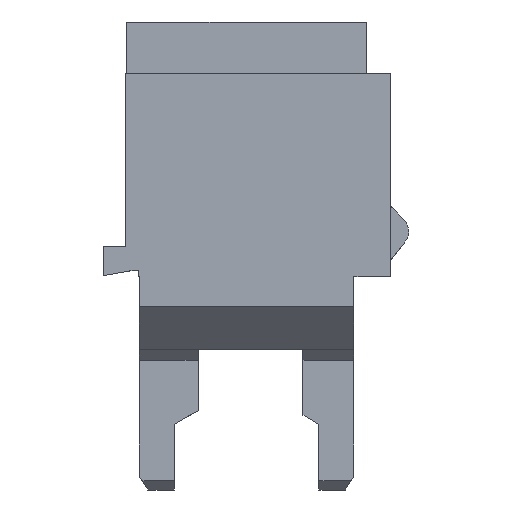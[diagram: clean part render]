
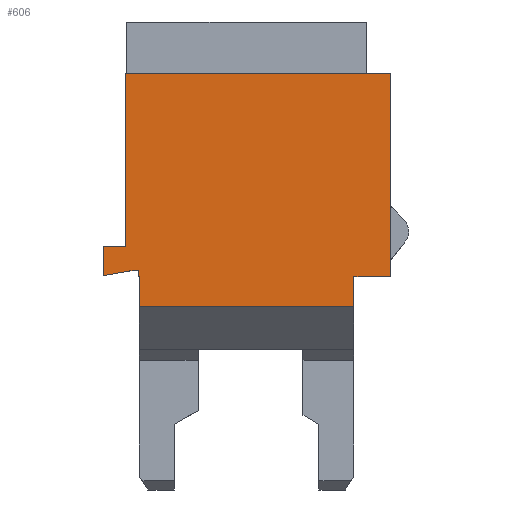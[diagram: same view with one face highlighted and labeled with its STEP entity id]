
A CAD part, left-side view. The second image highlights one B-rep face of the part: STEP entity #606.
In plain terms, the highlighted planar face has unit normal (-1, 0, 0).
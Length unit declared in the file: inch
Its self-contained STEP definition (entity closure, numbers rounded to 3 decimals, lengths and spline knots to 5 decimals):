
#606=ADVANCED_FACE('',(#1566),#1567,.T.);
#782=EDGE_CURVE('',#1823,#1816,#1826,.T.);
#816=EDGE_CURVE('',#1836,#1872,#1875,.T.);
#822=EDGE_CURVE('',#1880,#1872,#1883,.T.);
#858=EDGE_CURVE('',#1880,#1932,#1935,.T.);
#1100=EDGE_CURVE('',#2256,#2253,#2257,.T.);
#1106=EDGE_CURVE('',#2256,#2261,#2264,.T.);
#1136=EDGE_CURVE('',#2301,#1816,#2302,.T.);
#1138=EDGE_CURVE('',#2261,#1823,#2304,.T.);
#1140=EDGE_CURVE('',#2253,#2306,#2307,.T.);
#1142=EDGE_CURVE('',#2306,#2309,#2310,.T.);
#1144=EDGE_CURVE('',#2312,#2309,#2313,.T.);
#1146=EDGE_CURVE('',#1836,#2312,#2315,.T.);
#1148=EDGE_CURVE('',#2301,#1932,#2317,.T.);
#1566=FACE_OUTER_BOUND('',#2773,.T.);
#1567=PLANE('',#2774);
#1816=VERTEX_POINT('',#3138);
#1823=VERTEX_POINT('',#3149);
#1826=LINE('',#3154,#3155);
#1836=VERTEX_POINT('',#3169);
#1872=VERTEX_POINT('',#3227);
#1875=LINE('',#3232,#3233);
#1880=VERTEX_POINT('',#3241);
#1883=LINE('',#3246,#3247);
#1932=VERTEX_POINT('',#3327);
#1935=LINE('',#3332,#3333);
#2253=VERTEX_POINT('',#3877);
#2256=VERTEX_POINT('',#3882);
#2257=LINE('',#3883,#3884);
#2261=VERTEX_POINT('',#3891);
#2264=LINE('',#3896,#3897);
#2301=VERTEX_POINT('',#3962);
#2302=LINE('',#3963,#3964);
#2304=LINE('',#3967,#3968);
#2306=VERTEX_POINT('',#3971);
#2307=LINE('',#3972,#3973);
#2309=VERTEX_POINT('',#3976);
#2310=LINE('',#3977,#3978);
#2312=VERTEX_POINT('',#3981);
#2313=LINE('',#3982,#3983);
#2315=LINE('',#3986,#3987);
#2317=LINE('',#3990,#3991);
#2773=EDGE_LOOP('',(#5173,#5174,#5175,#5176,#5177,#5178,#5179,#5180,#5181,#5182,#5183,#5184,#5185));
#2774=AXIS2_PLACEMENT_3D('',#5186,#5187,#5188);
#3138=CARTESIAN_POINT('',(0.0,-0.0705,2.075));
#3149=CARTESIAN_POINT('',(0.0,1.4745,2.075));
#3154=CARTESIAN_POINT('',(0.0,-0.0555,2.075));
#3155=VECTOR('',#5633,0.03937);
#3169=CARTESIAN_POINT('',(0.0,1.395,0.89));
#3227=CARTESIAN_POINT('',(0.0,1.395,0.715));
#3232=CARTESIAN_POINT('',(0.0,1.395,0.71016));
#3233=VECTOR('',#5660,0.03937);
#3241=CARTESIAN_POINT('',(0.0,0.145,0.715));
#3246=CARTESIAN_POINT('',(0.0,1.614,0.715));
#3247=VECTOR('',#5663,0.03937);
#3327=CARTESIAN_POINT('',(0.0,0.145,0.89));
#3332=CARTESIAN_POINT('',(0.0,0.145,0.71016));
#3333=VECTOR('',#5685,0.03937);
#3877=CARTESIAN_POINT('',(0.0,1.6045,0.89553));
#3882=CARTESIAN_POINT('',(0.0,1.6045,1.068));
#3883=CARTESIAN_POINT('',(0.0,1.6045,1.44156));
#3884=VECTOR('',#5832,0.03937);
#3891=CARTESIAN_POINT('',(0.0,1.4745,1.068));
#3896=CARTESIAN_POINT('',(0.0,-0.00806,1.068));
#3897=VECTOR('',#5835,0.03937);
#3962=CARTESIAN_POINT('',(0.0,-0.0705,0.89));
#3963=CARTESIAN_POINT('',(0.0,-0.0705,1.45141));
#3964=VECTOR('',#5852,0.03937);
#3967=CARTESIAN_POINT('',(0.0,1.4745,1.19609));
#3968=VECTOR('',#5853,0.03937);
#3971=CARTESIAN_POINT('',(0.,1.44366,0.92389));
#3972=CARTESIAN_POINT('',(0.,0.72763,1.05014));
#3973=VECTOR('',#5854,0.03937);
#3976=CARTESIAN_POINT('',(0.,1.398,0.92389));
#3977=CARTESIAN_POINT('',(0.,1.44366,0.92389));
#3978=VECTOR('',#5855,0.03937);
#3981=CARTESIAN_POINT('',(0.0,1.398,0.89));
#3982=CARTESIAN_POINT('',(0.0,1.398,1.46125));
#3983=VECTOR('',#5856,0.03937);
#3986=CARTESIAN_POINT('',(0.0,1.6075,0.89));
#3987=VECTOR('',#5857,0.03937);
#3990=CARTESIAN_POINT('',(0.0,1.6075,0.89));
#3991=VECTOR('',#5858,0.03937);
#5173=ORIENTED_EDGE('',*,*,#1136,.T.);
#5174=ORIENTED_EDGE('',*,*,#782,.F.);
#5175=ORIENTED_EDGE('',*,*,#1138,.F.);
#5176=ORIENTED_EDGE('',*,*,#1106,.F.);
#5177=ORIENTED_EDGE('',*,*,#1100,.T.);
#5178=ORIENTED_EDGE('',*,*,#1140,.T.);
#5179=ORIENTED_EDGE('',*,*,#1142,.T.);
#5180=ORIENTED_EDGE('',*,*,#1144,.F.);
#5181=ORIENTED_EDGE('',*,*,#1146,.F.);
#5182=ORIENTED_EDGE('',*,*,#816,.T.);
#5183=ORIENTED_EDGE('',*,*,#822,.F.);
#5184=ORIENTED_EDGE('',*,*,#858,.T.);
#5185=ORIENTED_EDGE('',*,*,#1148,.F.);
#5186=CARTESIAN_POINT('',(0.0,-0.0555,1.4825));
#5187=DIRECTION('',(-1.0,0.0,0.0));
#5188=DIRECTION('',(0.0,0.0,-1.0));
#5633=DIRECTION('',(0.0,-1.0,0.0));
#5660=DIRECTION('',(-0.0,-0.0,-1.0));
#5663=DIRECTION('',(0.0,1.0,0.0));
#5685=DIRECTION('',(0.0,0.0,1.0));
#5832=DIRECTION('',(-0.0,-0.0,-1.0));
#5835=DIRECTION('',(-0.0,-1.0,-0.0));
#5852=DIRECTION('',(0.0,0.0,1.0));
#5853=DIRECTION('',(0.0,0.0,1.0));
#5854=DIRECTION('',(0.0,-0.985,0.174));
#5855=DIRECTION('',(0.0,-1.0,0.0));
#5856=DIRECTION('',(0.0,0.0,1.0));
#5857=DIRECTION('',(0.0,1.0,0.0));
#5858=DIRECTION('',(0.0,1.0,0.0));
